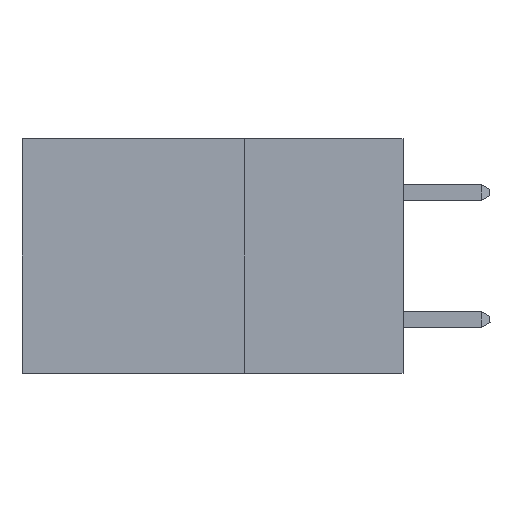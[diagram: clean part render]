
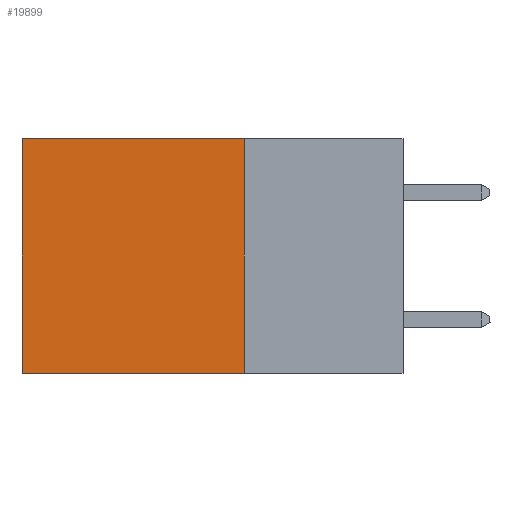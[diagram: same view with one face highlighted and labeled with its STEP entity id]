
A CAD part, left-side view. The second image highlights one B-rep face of the part: STEP entity #19899.
In plain terms, the highlighted planar face has unit normal (-1, 0, 0).
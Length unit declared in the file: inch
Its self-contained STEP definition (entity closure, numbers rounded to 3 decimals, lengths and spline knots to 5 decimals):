
#1548 = CARTESIAN_POINT ( 'NONE',  ( 0.2875, 0.25, 0. ) ) ;
#1714 = DIRECTION ( 'NONE',  ( 0., 0., -1. ) ) ;
#1748 = LINE ( 'NONE', #1548, #6956 ) ;
#2591 = CARTESIAN_POINT ( 'NONE',  ( 0.2875, 0.25, -0.37 ) ) ;
#3114 = CARTESIAN_POINT ( 'NONE',  ( 0.2875, 0.25, 0. ) ) ;
#3351 = VECTOR ( 'NONE', #19034, 39.37008 ) ;
#4292 = VECTOR ( 'NONE', #13681, 39.37008 ) ;
#4342 = LINE ( 'NONE', #10820, #3351 ) ;
#4636 = ORIENTED_EDGE ( 'NONE', *, *, #19382, .T. ) ;
#5764 = EDGE_LOOP ( 'NONE', ( #4636, #12430, #12478, #9562 ) ) ;
#6956 = VECTOR ( 'NONE', #17369, 39.37008 ) ;
#7196 = CARTESIAN_POINT ( 'NONE',  ( 0.2875, 0.25, -0.37 ) ) ;
#9510 = LINE ( 'NONE', #16036, #13222 ) ;
#9562 = ORIENTED_EDGE ( 'NONE', *, *, #11140, .T. ) ;
#9720 = PLANE ( 'NONE',  #19366 ) ;
#10820 = CARTESIAN_POINT ( 'NONE',  ( 0.2875, 0.6, 0. ) ) ;
#11140 = EDGE_CURVE ( 'NONE', #15218, #20758, #1748, .T. ) ;
#12430 = ORIENTED_EDGE ( 'NONE', *, *, #14205, .F. ) ;
#12478 = ORIENTED_EDGE ( 'NONE', *, *, #20250, .F. ) ;
#12914 = DIRECTION ( 'NONE',  ( 1., 0., 0. ) ) ;
#13222 = VECTOR ( 'NONE', #14406, 39.37008 ) ;
#13275 = LINE ( 'NONE', #7196, #4292 ) ;
#13681 = DIRECTION ( 'NONE',  ( 0., 1., 0. ) ) ;
#14205 = EDGE_CURVE ( 'NONE', #19990, #18923, #13275, .T. ) ;
#14406 = DIRECTION ( 'NONE',  ( 0., 0., -1. ) ) ;
#15218 = VERTEX_POINT ( 'NONE', #15902 ) ;
#15902 = CARTESIAN_POINT ( 'NONE',  ( 0.2875, 0.25, 0. ) ) ;
#16036 = CARTESIAN_POINT ( 'NONE',  ( 0.2875, 0.25, 0. ) ) ;
#16143 = FACE_OUTER_BOUND ( 'NONE', #5764, .T. ) ;
#17369 = DIRECTION ( 'NONE',  ( 0., 1., 0. ) ) ;
#18112 = CARTESIAN_POINT ( 'NONE',  ( 0.2875, 0.6, 0. ) ) ;
#18923 = VERTEX_POINT ( 'NONE', #20549 ) ;
#19034 = DIRECTION ( 'NONE',  ( 0., 0., -1. ) ) ;
#19366 = AXIS2_PLACEMENT_3D ( 'NONE', #3114, #12914, #1714 ) ;
#19382 = EDGE_CURVE ( 'NONE', #20758, #18923, #4342, .T. ) ;
#19899 = ADVANCED_FACE ( 'NONE', ( #16143 ), #9720, .F. ) ;
#19990 = VERTEX_POINT ( 'NONE', #2591 ) ;
#20250 = EDGE_CURVE ( 'NONE', #15218, #19990, #9510, .T. ) ;
#20549 = CARTESIAN_POINT ( 'NONE',  ( 0.2875, 0.6, -0.37 ) ) ;
#20758 = VERTEX_POINT ( 'NONE', #18112 ) ;
